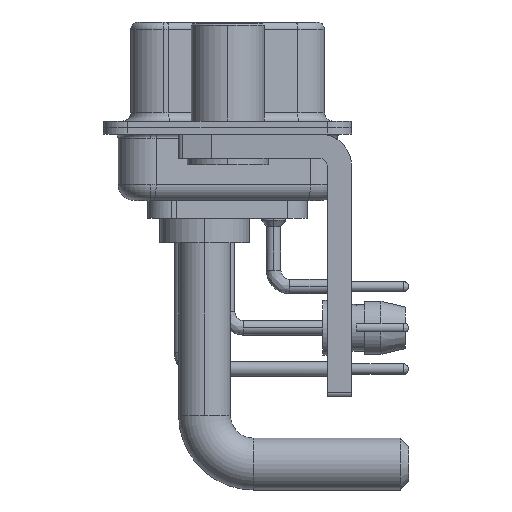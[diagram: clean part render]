
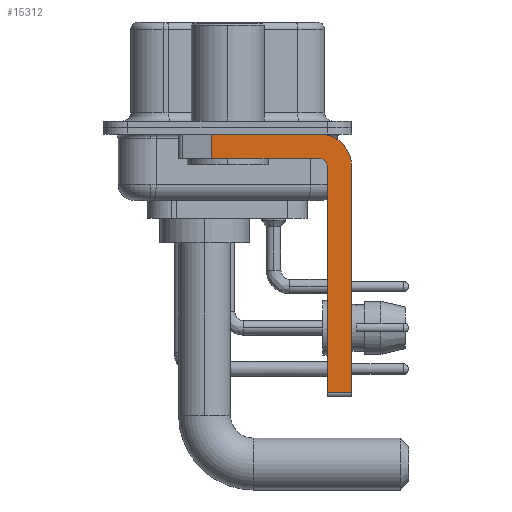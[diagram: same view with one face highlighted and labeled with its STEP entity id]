
A CAD part, left-side view. The second image highlights one B-rep face of the part: STEP entity #15312.
In plain terms, the highlighted planar face has unit normal (-1, 0, 0).
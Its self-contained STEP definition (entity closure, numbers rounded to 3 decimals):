
#53 = DIRECTION ( 'NONE',  ( 0., 1., 0. ) ) ;
#161 = EDGE_CURVE ( 'NONE', #21297, #30289, #20111, .T. ) ;
#763 = LINE ( 'NONE', #29988, #32409 ) ;
#1960 = EDGE_LOOP ( 'NONE', ( #32559, #12872, #5046, #13753, #8984, #6285, #33619, #17984 ) ) ;
#2103 = EDGE_CURVE ( 'NONE', #37511, #27872, #763, .T. ) ;
#2941 = CARTESIAN_POINT ( 'NONE',  ( -2.9, -5.65, -16.35 ) ) ;
#3109 = CARTESIAN_POINT ( 'NONE',  ( -2.9, -5.65, -1.9 ) ) ;
#4364 = CARTESIAN_POINT ( 'NONE',  ( -2.9, -6.15, -2.4 ) ) ;
#5046 = ORIENTED_EDGE ( 'NONE', *, *, #161, .F. ) ;
#5290 = AXIS2_PLACEMENT_3D ( 'NONE', #13415, #28288, #8417 ) ;
#5489 = CARTESIAN_POINT ( 'NONE',  ( -2.9, -5.65, -1.9 ) ) ;
#5565 = VERTEX_POINT ( 'NONE', #4364 ) ;
#5998 = DIRECTION ( 'NONE',  ( 0., 0., -1. ) ) ;
#6285 = ORIENTED_EDGE ( 'NONE', *, *, #36705, .T. ) ;
#6327 = VERTEX_POINT ( 'NONE', #21253 ) ;
#7591 = CARTESIAN_POINT ( 'NONE',  ( -2.9, -7.65, -16.35 ) ) ;
#7606 = EDGE_CURVE ( 'NONE', #5565, #21297, #36165, .T. ) ;
#7714 = CARTESIAN_POINT ( 'NONE',  ( -2.9, -6.15, -16.6 ) ) ;
#8190 = VECTOR ( 'NONE', #53, 1000. ) ;
#8201 = CARTESIAN_POINT ( 'NONE',  ( -2.9, -7.65, -2.4 ) ) ;
#8417 = DIRECTION ( 'NONE',  ( 0., 0., -1. ) ) ;
#8665 = VERTEX_POINT ( 'NONE', #16721 ) ;
#8848 = DIRECTION ( 'NONE',  ( 1., 0., 0. ) ) ;
#8984 = ORIENTED_EDGE ( 'NONE', *, *, #36036, .F. ) ;
#9042 = PLANE ( 'NONE',  #28061 ) ;
#9547 = VERTEX_POINT ( 'NONE', #30875 ) ;
#9698 = EDGE_CURVE ( 'NONE', #9547, #30289, #28946, .T. ) ;
#10598 = EDGE_CURVE ( 'NONE', #6327, #37511, #24178, .T. ) ;
#11970 = VECTOR ( 'NONE', #34649, 1000. ) ;
#12872 = ORIENTED_EDGE ( 'NONE', *, *, #9698, .T. ) ;
#13415 = CARTESIAN_POINT ( 'NONE',  ( -2.9, -5.65, -2.4 ) ) ;
#13468 = DIRECTION ( 'NONE',  ( 0., -1., 0. ) ) ;
#13753 = ORIENTED_EDGE ( 'NONE', *, *, #7606, .F. ) ;
#14214 = LINE ( 'NONE', #7714, #11970 ) ;
#15294 = CARTESIAN_POINT ( 'NONE',  ( -2.9, 0.978, -1.9 ) ) ;
#15312 = ADVANCED_FACE ( 'NONE', ( #20137 ), #9042, .F. ) ;
#16331 = LINE ( 'NONE', #30653, #21165 ) ;
#16721 = CARTESIAN_POINT ( 'NONE',  ( -2.9, -6.15, -16.35 ) ) ;
#17119 = CARTESIAN_POINT ( 'NONE',  ( -2.9, -5.65, -2.4 ) ) ;
#17984 = ORIENTED_EDGE ( 'NONE', *, *, #10598, .F. ) ;
#20111 = LINE ( 'NONE', #3109, #8190 ) ;
#20137 = FACE_OUTER_BOUND ( 'NONE', #1960, .T. ) ;
#21165 = VECTOR ( 'NONE', #13468, 1000. ) ;
#21253 = CARTESIAN_POINT ( 'NONE',  ( -2.9, -5.65, -0.4 ) ) ;
#21297 = VERTEX_POINT ( 'NONE', #5489 ) ;
#24075 = DIRECTION ( 'NONE',  ( 0., 0., -1. ) ) ;
#24178 = CIRCLE ( 'NONE', #5290, 2. ) ;
#25936 = VECTOR ( 'NONE', #37732, 1000. ) ;
#26082 = CARTESIAN_POINT ( 'NONE',  ( -2.9, 0.978, -1.9 ) ) ;
#26430 = LINE ( 'NONE', #2941, #30916 ) ;
#27872 = VERTEX_POINT ( 'NONE', #7591 ) ;
#28061 = AXIS2_PLACEMENT_3D ( 'NONE', #35027, #8848, #5998 ) ;
#28288 = DIRECTION ( 'NONE',  ( 1., 0., 0. ) ) ;
#28375 = DIRECTION ( 'NONE',  ( 0., 0., 1. ) ) ;
#28757 = DIRECTION ( 'NONE',  ( -1., 0., 0. ) ) ;
#28946 = LINE ( 'NONE', #26082, #25936 ) ;
#29988 = CARTESIAN_POINT ( 'NONE',  ( -2.9, -7.65, -2.4 ) ) ;
#30289 = VERTEX_POINT ( 'NONE', #15294 ) ;
#30653 = CARTESIAN_POINT ( 'NONE',  ( -2.9, 3., -0.4 ) ) ;
#30875 = CARTESIAN_POINT ( 'NONE',  ( -2.9, 0.978, -0.4 ) ) ;
#30916 = VECTOR ( 'NONE', #32544, 1000. ) ;
#32409 = VECTOR ( 'NONE', #24075, 1000. ) ;
#32544 = DIRECTION ( 'NONE',  ( 0., -1., 0. ) ) ;
#32559 = ORIENTED_EDGE ( 'NONE', *, *, #36466, .F. ) ;
#33619 = ORIENTED_EDGE ( 'NONE', *, *, #2103, .F. ) ;
#34649 = DIRECTION ( 'NONE',  ( 0., 0., 1. ) ) ;
#35027 = CARTESIAN_POINT ( 'NONE',  ( -2.9, -5.65, -2.4 ) ) ;
#36036 = EDGE_CURVE ( 'NONE', #8665, #5565, #14214, .T. ) ;
#36165 = CIRCLE ( 'NONE', #37376, 0.5 ) ;
#36466 = EDGE_CURVE ( 'NONE', #9547, #6327, #16331, .T. ) ;
#36705 = EDGE_CURVE ( 'NONE', #8665, #27872, #26430, .T. ) ;
#37376 = AXIS2_PLACEMENT_3D ( 'NONE', #17119, #28757, #28375 ) ;
#37511 = VERTEX_POINT ( 'NONE', #8201 ) ;
#37732 = DIRECTION ( 'NONE',  ( 0., 0., -1. ) ) ;
